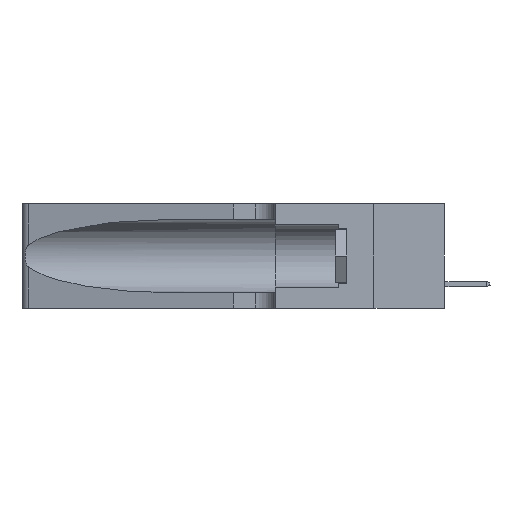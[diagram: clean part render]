
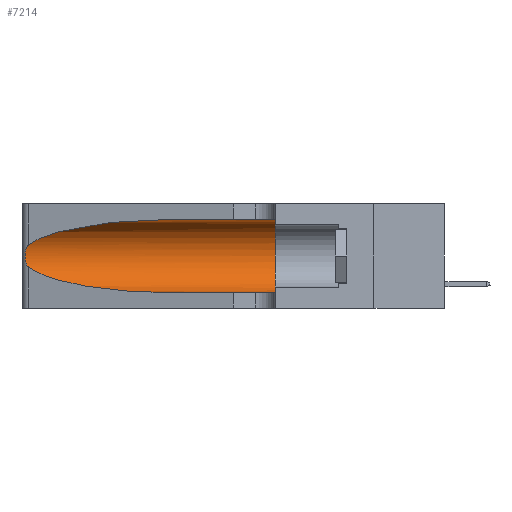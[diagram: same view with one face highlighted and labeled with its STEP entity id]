
A CAD part, left-side view. The second image highlights one B-rep face of the part: STEP entity #7214.
In plain terms, the highlighted cylindrical face has radius 3.308 mm (diameter 6.617 mm), a partial arc.
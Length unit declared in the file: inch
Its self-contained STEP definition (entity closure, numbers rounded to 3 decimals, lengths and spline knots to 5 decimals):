
#361 = VECTOR ( 'NONE', #2925, 39.37008 ) ;
#779 = CARTESIAN_POINT ( 'NONE',  ( 0.25854, 1.2359, 0.20912 ) ) ;
#1069 = CARTESIAN_POINT ( 'NONE',  ( 0.25639, 1.23184, 0.21858 ) ) ;
#1378 = CARTESIAN_POINT ( 'NONE',  ( 0.1305, 0.35, 0.31525 ) ) ;
#1606 = VERTEX_POINT ( 'NONE', #17939 ) ;
#1727 = B_SPLINE_CURVE_WITH_KNOTS ( 'NONE', 3,
 ( #15018, #18340, #1069, #4532, #779, #11273, #21871, #2835, #15093, #4385, #20028, #9528, #21796, #2536 ),
 .UNSPECIFIED., .F., .F.,
 ( 4, 2, 2, 2, 2, 2, 4 ),
 ( 0., 0.00027, 0.00053, 0.00107, 0.0016, 0.00187, 0.00214 ),
 .UNSPECIFIED. ) ;
#1881 = DIRECTION ( 'NONE',  ( 0., 0., 1. ) ) ;
#2522 = LINE ( 'NONE', #15109, #4992 ) ;
#2536 = CARTESIAN_POINT ( 'NONE',  ( 0.25487, 1.22718, 0.14631 ) ) ;
#2835 = CARTESIAN_POINT ( 'NONE',  ( 0.26075, 1.23896, 0.178 ) ) ;
#2895 = EDGE_CURVE ( 'NONE', #11204, #1606, #11870, .T. ) ;
#2925 = DIRECTION ( 'NONE',  ( 0., -1., 0. ) ) ;
#3062 = CIRCLE ( 'NONE', #22580, 0.13025 ) ;
#3321 = VERTEX_POINT ( 'NONE', #1378 ) ;
#3968 = AXIS2_PLACEMENT_3D ( 'NONE', #21722, #14484, #19796 ) ;
#4385 = CARTESIAN_POINT ( 'NONE',  ( 0.25856, 1.23593, 0.16098 ) ) ;
#4532 = CARTESIAN_POINT ( 'NONE',  ( 0.25787, 1.23484, 0.2124 ) ) ;
#4992 = VECTOR ( 'NONE', #22166, 39.37008 ) ;
#5298 = ORIENTED_EDGE ( 'NONE', *, *, #19534, .T. ) ;
#5862 =( BOUNDED_CURVE ( )  B_SPLINE_CURVE ( 3, ( #14063, #6960, #17620, #21145 ),
 .UNSPECIFIED., .F., .F. ) 
 B_SPLINE_CURVE_WITH_KNOTS ( ( 4, 4 ),
 ( 3.44316, 4.71239 ),
 .UNSPECIFIED. ) 
 CURVE ( )  GEOMETRIC_REPRESENTATION_ITEM ( )  RATIONAL_B_SPLINE_CURVE ( ( 1., 0.87, 0.87, 1. ) ) 
 REPRESENTATION_ITEM ( '' )  );
#6448 = VERTEX_POINT ( 'NONE', #10834 ) ;
#6729 = ORIENTED_EDGE ( 'NONE', *, *, #17881, .T. ) ;
#6960 = CARTESIAN_POINT ( 'NONE',  ( 0.2373, 1.15595, 0.08982 ) ) ;
#7150 = CARTESIAN_POINT ( 'NONE',  ( 0.25487, 1.22718, 0.22369 ) ) ;
#7214 = ADVANCED_FACE ( 'NONE', ( #9704 ), #15411, .F. ) ;
#8454 = CARTESIAN_POINT ( 'NONE',  ( 0.1305, 0.72297, 0.31525 ) ) ;
#9075 = CARTESIAN_POINT ( 'NONE',  ( 0.1305, 0.72297, 0.05475 ) ) ;
#9528 = CARTESIAN_POINT ( 'NONE',  ( 0.25639, 1.23186, 0.15144 ) ) ;
#9704 = FACE_OUTER_BOUND ( 'NONE', #10512, .T. ) ;
#9963 = ORIENTED_EDGE ( 'NONE', *, *, #2895, .T. ) ;
#10275 = CARTESIAN_POINT ( 'NONE',  ( 0.18966, 0.96281, 0.31525 ) ) ;
#10512 = EDGE_LOOP ( 'NONE', ( #6729, #10925, #5298, #9963, #19097, #13269 ) ) ;
#10709 = CARTESIAN_POINT ( 'NONE',  ( 0.1305, 0.35, 0.185 ) ) ;
#10834 = CARTESIAN_POINT ( 'NONE',  ( 0.1305, 0.72297, 0.31525 ) ) ;
#10925 = ORIENTED_EDGE ( 'NONE', *, *, #20476, .T. ) ;
#11204 = VERTEX_POINT ( 'NONE', #9075 ) ;
#11273 = CARTESIAN_POINT ( 'NONE',  ( 0.26018, 1.23835, 0.19895 ) ) ;
#11870 = LINE ( 'NONE', #20625, #361 ) ;
#12442 = DIRECTION ( 'NONE',  ( 0., 1., 0. ) ) ;
#13269 = ORIENTED_EDGE ( 'NONE', *, *, #14710, .F. ) ;
#13947 = VERTEX_POINT ( 'NONE', #18619 ) ;
#14063 = CARTESIAN_POINT ( 'NONE',  ( 0.25487, 1.22718, 0.14631 ) ) ;
#14266 = CARTESIAN_POINT ( 'NONE',  ( 0.2373, 1.15595, 0.28018 ) ) ;
#14484 = DIRECTION ( 'NONE',  ( 0., -1., 0. ) ) ;
#14710 = EDGE_CURVE ( 'NONE', #6448, #3321, #2522, .T. ) ;
#15018 = CARTESIAN_POINT ( 'NONE',  ( 0.25487, 1.22718, 0.22369 ) ) ;
#15093 = CARTESIAN_POINT ( 'NONE',  ( 0.26017, 1.23833, 0.17102 ) ) ;
#15109 = CARTESIAN_POINT ( 'NONE',  ( 0.1305, 1.61858, 0.31525 ) ) ;
#15358 = VERTEX_POINT ( 'NONE', #19426 ) ;
#15411 = CYLINDRICAL_SURFACE ( 'NONE', #3968, 0.13025 ) ;
#17620 = CARTESIAN_POINT ( 'NONE',  ( 0.18966, 0.96281, 0.05475 ) ) ;
#17881 = EDGE_CURVE ( 'NONE', #6448, #13947, #22139, .T. ) ;
#17939 = CARTESIAN_POINT ( 'NONE',  ( 0.1305, 0.35, 0.05475 ) ) ;
#18238 = EDGE_CURVE ( 'NONE', #3321, #1606, #3062, .T. ) ;
#18340 = CARTESIAN_POINT ( 'NONE',  ( 0.25555, 1.22994, 0.2215 ) ) ;
#18619 = CARTESIAN_POINT ( 'NONE',  ( 0.25487, 1.22718, 0.22369 ) ) ;
#19097 = ORIENTED_EDGE ( 'NONE', *, *, #18238, .F. ) ;
#19426 = CARTESIAN_POINT ( 'NONE',  ( 0.25487, 1.22718, 0.14631 ) ) ;
#19534 = EDGE_CURVE ( 'NONE', #15358, #11204, #5862, .T. ) ;
#19796 = DIRECTION ( 'NONE',  ( 0., 0., -1. ) ) ;
#20028 = CARTESIAN_POINT ( 'NONE',  ( 0.25789, 1.23486, 0.15765 ) ) ;
#20476 = EDGE_CURVE ( 'NONE', #13947, #15358, #1727, .T. ) ;
#20625 = CARTESIAN_POINT ( 'NONE',  ( 0.1305, 1.61858, 0.05475 ) ) ;
#21145 = CARTESIAN_POINT ( 'NONE',  ( 0.1305, 0.72297, 0.05475 ) ) ;
#21722 = CARTESIAN_POINT ( 'NONE',  ( 0.1305, 1.61858, 0.185 ) ) ;
#21796 = CARTESIAN_POINT ( 'NONE',  ( 0.25555, 1.22993, 0.14849 ) ) ;
#21871 = CARTESIAN_POINT ( 'NONE',  ( 0.26075, 1.23896, 0.19203 ) ) ;
#22139 =( BOUNDED_CURVE ( )  B_SPLINE_CURVE ( 3, ( #8454, #10275, #14266, #7150 ),
 .UNSPECIFIED., .F., .F. ) 
 B_SPLINE_CURVE_WITH_KNOTS ( ( 4, 4 ),
 ( 1.5708, 2.84003 ),
 .UNSPECIFIED. ) 
 CURVE ( )  GEOMETRIC_REPRESENTATION_ITEM ( )  RATIONAL_B_SPLINE_CURVE ( ( 1., 0.87, 0.87, 1. ) ) 
 REPRESENTATION_ITEM ( '' )  );
#22166 = DIRECTION ( 'NONE',  ( 0., -1., 0. ) ) ;
#22580 = AXIS2_PLACEMENT_3D ( 'NONE', #10709, #12442, #1881 ) ;
